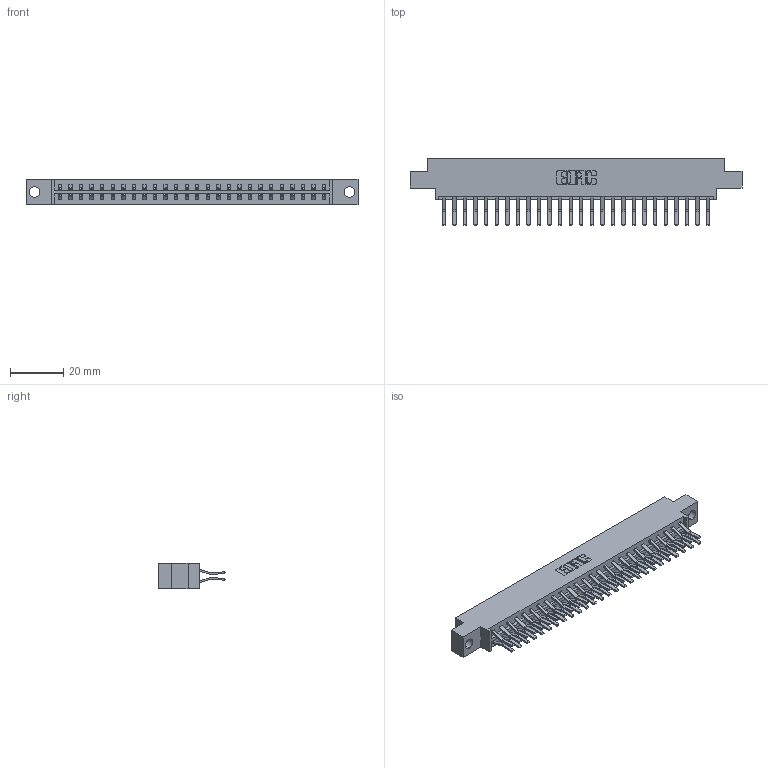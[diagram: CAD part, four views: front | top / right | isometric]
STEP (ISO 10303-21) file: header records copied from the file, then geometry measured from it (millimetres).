
FILE_DESCRIPTION (( 'STEP AP203' ), '1' );
FILE_NAME ('333-052-560-804.STEP', '2018-08-04T03:23:01', ( '' ), ( '' ), 'SwSTEP 2.0', 'SolidWorks 2016', '' );
FILE_SCHEMA (( 'CONFIG_CONTROL_DESIGN' ));
Length unit declared in the file: inch
Products named in the file (3): 333 Part_Offset - .156 Dia - TH; 345-292-001_560 Tail; 333-052-560-804
Assembly tree (53 placements, depth 2):
  333-052-560-804
    333 Part_Offset - .156 Dia - TH
    345-292-001_560 Tail  x52
Bounding box: 124.56 x 24.78 x 9.4 mm (x, y, z)
Volume: 12592.6 mm3; surface area: 15708.2 mm2
Topology: 53 solids, 53 shells, 2926 faces, 8695 edges, 5726 vertices
Faces by surface type: plane 1946, cylinder 980
Entity records: 19019 total; most frequent: CARTESIAN_POINT 3174, ORIENTED_EDGE 3110, DIRECTION 2743, EDGE_CURVE 1555, VECTOR 1423, LINE 1423, VERTEX_POINT 1034, AXIS2_PLACEMENT_3D 660
